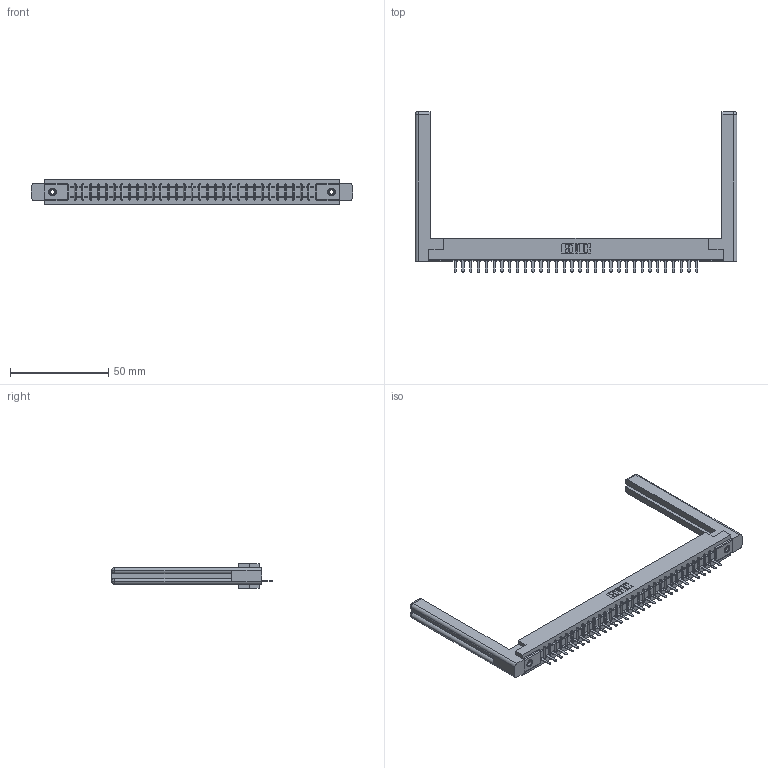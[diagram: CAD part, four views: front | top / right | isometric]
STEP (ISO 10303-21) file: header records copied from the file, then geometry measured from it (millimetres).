
FILE_DESCRIPTION (( 'STEP AP203' ), '1' );
FILE_NAME ('307-032-521-158.STEP', '2019-09-05T05:18:03', ( '' ), ( '' ), 'SwSTEP 2.0', 'SolidWorks 2016', '' );
FILE_SCHEMA (( 'CONFIG_CONTROL_DESIGN' ));
Length unit declared in the file: inch
Products named in the file (5): 307-220-058; 345-250-001_345-250-001-102; 307-290-002_521; 307-032-521-158; 307 Part_.156 Dia Mounting Holes
Assembly tree (37 placements, depth 2):
  307-032-521-158
    307 Part_.156 Dia Mounting Holes
    307-290-002_521  x32
    307-220-058  x2
    345-250-001_345-250-001-102  x2
Bounding box: 163.42 x 81.74 x 12.7 mm (x, y, z)
Volume: 24535.9 mm3; surface area: 26516 mm2
Topology: 37 solids, 37 shells, 2661 faces, 8101 edges, 5298 vertices
Faces by surface type: plane 1594, cylinder 977, sphere 66, torus 12, cone 12
Entity records: 32017 total; most frequent: CARTESIAN_POINT 5407, ORIENTED_EDGE 5336, DIRECTION 5218, EDGE_CURVE 2668, LINE 2036, VECTOR 2036, VERTEX_POINT 1726, AXIS2_PLACEMENT_3D 1591
